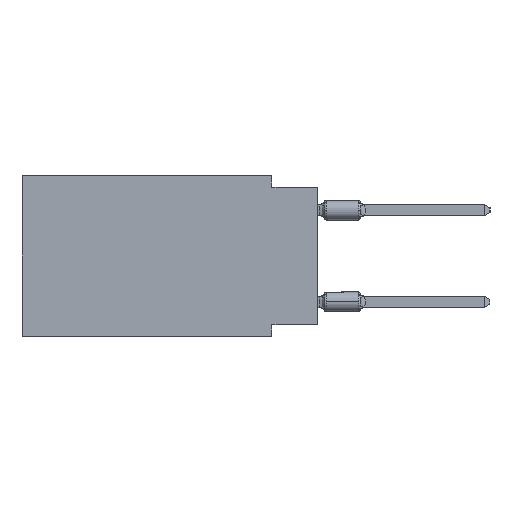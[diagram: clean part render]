
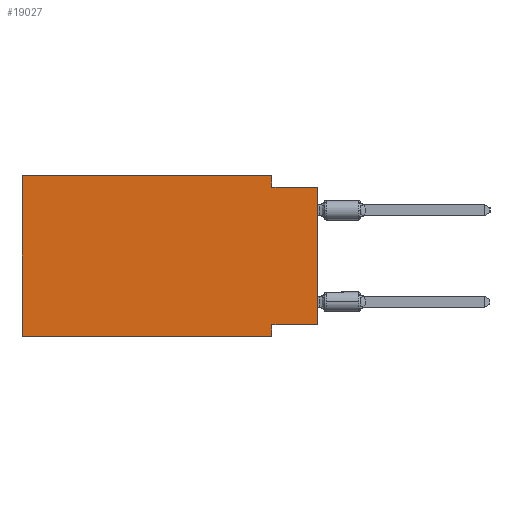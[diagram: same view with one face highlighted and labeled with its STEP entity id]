
A CAD part, left-side view. The second image highlights one B-rep face of the part: STEP entity #19027.
In plain terms, the highlighted planar face has unit normal (-1, 0, 0).
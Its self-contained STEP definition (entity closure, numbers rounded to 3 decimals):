
#204 = DIRECTION ( 'NONE',  ( 0., 0., 1. ) ) ;
#372 = DIRECTION ( 'NONE',  ( 0., 0., -1. ) ) ;
#3218 = VERTEX_POINT ( 'NONE', #61445 ) ;
#6888 = DIRECTION ( 'NONE',  ( 0., -1., 0. ) ) ;
#7668 = LINE ( 'NONE', #59237, #44408 ) ;
#7771 = VERTEX_POINT ( 'NONE', #62032 ) ;
#9386 = ORIENTED_EDGE ( 'NONE', *, *, #27751, .F. ) ;
#10055 = DIRECTION ( 'NONE',  ( 0., 1., 0. ) ) ;
#10557 = LINE ( 'NONE', #40210, #57014 ) ;
#11001 = VERTEX_POINT ( 'NONE', #13344 ) ;
#12188 = ORIENTED_EDGE ( 'NONE', *, *, #37985, .F. ) ;
#12541 = DIRECTION ( 'NONE',  ( 0., 0., -1. ) ) ;
#12848 = CARTESIAN_POINT ( 'NONE',  ( 0., 16.383, 0. ) ) ;
#13344 = CARTESIAN_POINT ( 'NONE',  ( 0., 2.54, 0. ) ) ;
#14312 = ORIENTED_EDGE ( 'NONE', *, *, #31799, .F. ) ;
#14321 = VECTOR ( 'NONE', #18144, 1000. ) ;
#17212 = EDGE_CURVE ( 'NONE', #32710, #58620, #7668, .T. ) ;
#17865 = LINE ( 'NONE', #23171, #58474 ) ;
#17994 = DIRECTION ( 'NONE',  ( 0., 0., 1. ) ) ;
#18144 = DIRECTION ( 'NONE',  ( 0., -1., 0. ) ) ;
#18331 = VECTOR ( 'NONE', #6888, 1000. ) ;
#18511 = CARTESIAN_POINT ( 'NONE',  ( 0., 16.383, -8.89 ) ) ;
#18938 = ORIENTED_EDGE ( 'NONE', *, *, #52000, .T. ) ;
#19027 = ADVANCED_FACE ( 'NONE', ( #50949 ), #26320, .F. ) ;
#20669 = LINE ( 'NONE', #35636, #47115 ) ;
#21795 = EDGE_CURVE ( 'NONE', #30847, #3218, #17865, .T. ) ;
#22778 = VECTOR ( 'NONE', #10055, 1000. ) ;
#23171 = CARTESIAN_POINT ( 'NONE',  ( 0., 2.54, -8.89 ) ) ;
#23291 = AXIS2_PLACEMENT_3D ( 'NONE', #35964, #56255, #56573 ) ;
#24496 = LINE ( 'NONE', #45784, #49246 ) ;
#26320 = PLANE ( 'NONE',  #23291 ) ;
#27523 = LINE ( 'NONE', #12848, #18331 ) ;
#27751 = EDGE_CURVE ( 'NONE', #11001, #61678, #20669, .T. ) ;
#30732 = CARTESIAN_POINT ( 'NONE',  ( 0., 0., -0.635 ) ) ;
#30847 = VERTEX_POINT ( 'NONE', #59849 ) ;
#31799 = EDGE_CURVE ( 'NONE', #7771, #11001, #27523, .T. ) ;
#31882 = VERTEX_POINT ( 'NONE', #18511 ) ;
#32710 = VERTEX_POINT ( 'NONE', #46196 ) ;
#33233 = ORIENTED_EDGE ( 'NONE', *, *, #17212, .T. ) ;
#34141 = ORIENTED_EDGE ( 'NONE', *, *, #53974, .F. ) ;
#34801 = EDGE_CURVE ( 'NONE', #31882, #7771, #24496, .T. ) ;
#35636 = CARTESIAN_POINT ( 'NONE',  ( 0., 2.54, 0. ) ) ;
#35964 = CARTESIAN_POINT ( 'NONE',  ( 0., 16.383, 0. ) ) ;
#37985 = EDGE_CURVE ( 'NONE', #61678, #58620, #10557, .T. ) ;
#40210 = CARTESIAN_POINT ( 'NONE',  ( 0., 0., -0.635 ) ) ;
#41000 = CARTESIAN_POINT ( 'NONE',  ( 0., 0., -8.255 ) ) ;
#41181 = DIRECTION ( 'NONE',  ( 0., -1., 0. ) ) ;
#44408 = VECTOR ( 'NONE', #17994, 1000. ) ;
#45784 = CARTESIAN_POINT ( 'NONE',  ( 0., 16.383, 0. ) ) ;
#46196 = CARTESIAN_POINT ( 'NONE',  ( 0., 0., -8.255 ) ) ;
#47115 = VECTOR ( 'NONE', #372, 1000. ) ;
#49246 = VECTOR ( 'NONE', #204, 1000. ) ;
#50949 = FACE_OUTER_BOUND ( 'NONE', #59490, .T. ) ;
#52000 = EDGE_CURVE ( 'NONE', #31882, #3218, #58082, .T. ) ;
#53974 = EDGE_CURVE ( 'NONE', #32710, #30847, #60956, .T. ) ;
#54009 = CARTESIAN_POINT ( 'NONE',  ( 0., 2.54, -0.635 ) ) ;
#55562 = ORIENTED_EDGE ( 'NONE', *, *, #34801, .F. ) ;
#56255 = DIRECTION ( 'NONE',  ( 1., 0., 0. ) ) ;
#56573 = DIRECTION ( 'NONE',  ( 0., 0., -1. ) ) ;
#57014 = VECTOR ( 'NONE', #41181, 1000. ) ;
#58082 = LINE ( 'NONE', #62748, #14321 ) ;
#58474 = VECTOR ( 'NONE', #12541, 1000. ) ;
#58620 = VERTEX_POINT ( 'NONE', #30732 ) ;
#59237 = CARTESIAN_POINT ( 'NONE',  ( 0., 0., 0. ) ) ;
#59490 = EDGE_LOOP ( 'NONE', ( #33233, #12188, #9386, #14312, #55562, #18938, #65636, #34141 ) ) ;
#59849 = CARTESIAN_POINT ( 'NONE',  ( 0., 2.54, -8.255 ) ) ;
#60956 = LINE ( 'NONE', #41000, #22778 ) ;
#61445 = CARTESIAN_POINT ( 'NONE',  ( 0., 2.54, -8.89 ) ) ;
#61678 = VERTEX_POINT ( 'NONE', #54009 ) ;
#62032 = CARTESIAN_POINT ( 'NONE',  ( 0., 16.383, 0. ) ) ;
#62748 = CARTESIAN_POINT ( 'NONE',  ( 0., 16.383, -8.89 ) ) ;
#65636 = ORIENTED_EDGE ( 'NONE', *, *, #21795, .F. ) ;
